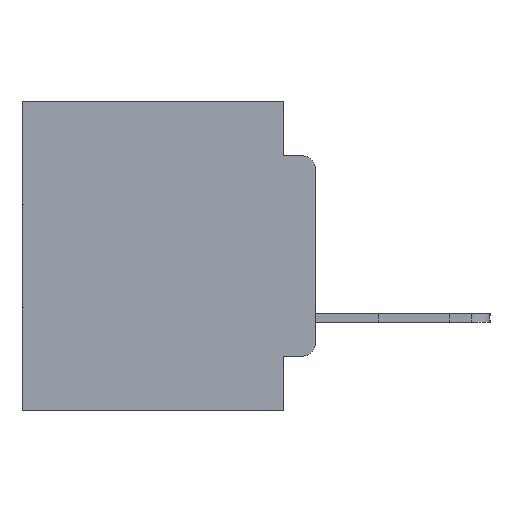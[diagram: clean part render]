
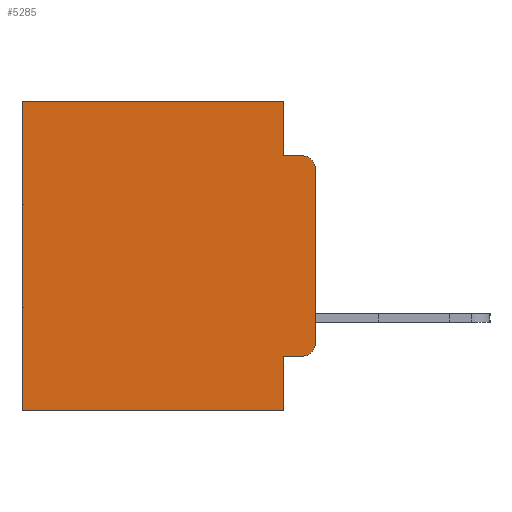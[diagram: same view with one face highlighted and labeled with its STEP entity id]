
A CAD part, left-side view. The second image highlights one B-rep face of the part: STEP entity #5285.
In plain terms, the highlighted planar face has unit normal (-1, 0, 0).
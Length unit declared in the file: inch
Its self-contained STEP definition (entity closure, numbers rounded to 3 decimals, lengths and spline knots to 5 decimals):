
#695 = VECTOR ( 'NONE', #17822, 39.37008 ) ;
#1607 = VERTEX_POINT ( 'NONE', #16577 ) ;
#1611 = CARTESIAN_POINT ( 'NONE',  ( 0.298, 0., 0. ) ) ;
#1712 = CARTESIAN_POINT ( 'NONE',  ( 0.298, 0., 0. ) ) ;
#1968 = LINE ( 'NONE', #10128, #19209 ) ;
#2167 = AXIS2_PLACEMENT_3D ( 'NONE', #1712, #5788, #24165 ) ;
#2727 = CARTESIAN_POINT ( 'NONE',  ( 0.298, 0.02, -0.3915 ) ) ;
#2819 = EDGE_CURVE ( 'NONE', #10604, #18837, #4257, .T. ) ;
#2824 = VERTEX_POINT ( 'NONE', #26158 ) ;
#3047 = CARTESIAN_POINT ( 'NONE',  ( 0.298, 0.051, -0.0885 ) ) ;
#3328 = ORIENTED_EDGE ( 'NONE', *, *, #24447, .F. ) ;
#3439 = VERTEX_POINT ( 'NONE', #17185 ) ;
#4044 = ORIENTED_EDGE ( 'NONE', *, *, #14340, .T. ) ;
#4171 = VERTEX_POINT ( 'NONE', #11172 ) ;
#4222 = FACE_OUTER_BOUND ( 'NONE', #17261, .T. ) ;
#4257 = LINE ( 'NONE', #1611, #21324 ) ;
#4798 = CARTESIAN_POINT ( 'NONE',  ( 0.298, 0.051, 0. ) ) ;
#5040 = DIRECTION ( 'NONE',  ( 0., 0., -1. ) ) ;
#5285 = ADVANCED_FACE ( 'NONE', ( #4222 ), #24320, .F. ) ;
#5398 = CARTESIAN_POINT ( 'NONE',  ( 0.298, 0., -0.1085 ) ) ;
#5788 = DIRECTION ( 'NONE',  ( 1., 0., 0. ) ) ;
#5996 = CIRCLE ( 'NONE', #6770, 0.02 ) ;
#6364 = DIRECTION ( 'NONE',  ( 0., 0., -1. ) ) ;
#6633 = DIRECTION ( 'NONE',  ( -1., 0., 0. ) ) ;
#6770 = AXIS2_PLACEMENT_3D ( 'NONE', #2727, #18402, #5040 ) ;
#7661 = DIRECTION ( 'NONE',  ( 0., -1., 0. ) ) ;
#8198 = DIRECTION ( 'NONE',  ( 0., 0., -1. ) ) ;
#9285 = VERTEX_POINT ( 'NONE', #15529 ) ;
#9409 = CARTESIAN_POINT ( 'NONE',  ( 0.298, 0.473, 0. ) ) ;
#10128 = CARTESIAN_POINT ( 'NONE',  ( 0.298, 0., 0. ) ) ;
#10375 = ORIENTED_EDGE ( 'NONE', *, *, #12024, .F. ) ;
#10604 = VERTEX_POINT ( 'NONE', #4798 ) ;
#10689 = VERTEX_POINT ( 'NONE', #5398 ) ;
#10917 = DIRECTION ( 'NONE',  ( 0., 1., 0. ) ) ;
#11079 = ORIENTED_EDGE ( 'NONE', *, *, #24829, .F. ) ;
#11172 = CARTESIAN_POINT ( 'NONE',  ( 0.298, 0.051, -0.5 ) ) ;
#11578 = LINE ( 'NONE', #18647, #16091 ) ;
#12024 = EDGE_CURVE ( 'NONE', #10689, #16149, #1968, .T. ) ;
#12135 = LINE ( 'NONE', #13140, #16666 ) ;
#12401 = DIRECTION ( 'NONE',  ( 0., 0., -1. ) ) ;
#12491 = ORIENTED_EDGE ( 'NONE', *, *, #18992, .F. ) ;
#12749 = CARTESIAN_POINT ( 'NONE',  ( 0.298, 0., -0.3915 ) ) ;
#13140 = CARTESIAN_POINT ( 'NONE',  ( 0.298, 0., -0.5 ) ) ;
#13609 = EDGE_CURVE ( 'NONE', #1607, #16149, #5996, .T. ) ;
#14340 = EDGE_CURVE ( 'NONE', #2824, #1607, #11578, .T. ) ;
#14456 = LINE ( 'NONE', #21890, #25434 ) ;
#14567 = ORIENTED_EDGE ( 'NONE', *, *, #17510, .T. ) ;
#15175 = DIRECTION ( 'NONE',  ( 0., 1., 0. ) ) ;
#15529 = CARTESIAN_POINT ( 'NONE',  ( 0.298, 0.02, -0.0885 ) ) ;
#15608 = CARTESIAN_POINT ( 'NONE',  ( 0.298, 0.473, 0. ) ) ;
#16091 = VECTOR ( 'NONE', #20752, 39.37008 ) ;
#16149 = VERTEX_POINT ( 'NONE', #12749 ) ;
#16319 = ORIENTED_EDGE ( 'NONE', *, *, #21419, .T. ) ;
#16577 = CARTESIAN_POINT ( 'NONE',  ( 0.298, 0.02, -0.4115 ) ) ;
#16666 = VECTOR ( 'NONE', #10917, 39.37008 ) ;
#16837 = CIRCLE ( 'NONE', #24294, 0.02 ) ;
#17185 = CARTESIAN_POINT ( 'NONE',  ( 0.298, 0.051, -0.0885 ) ) ;
#17261 = EDGE_LOOP ( 'NONE', ( #10375, #16319, #11079, #12491, #19062, #14567, #3328, #26865, #4044, #27561 ) ) ;
#17510 = EDGE_CURVE ( 'NONE', #18837, #26574, #23807, .T. ) ;
#17822 = DIRECTION ( 'NONE',  ( 0., 0., -1. ) ) ;
#17885 = EDGE_CURVE ( 'NONE', #2824, #4171, #27167, .T. ) ;
#18402 = DIRECTION ( 'NONE',  ( -1., 0., 0. ) ) ;
#18647 = CARTESIAN_POINT ( 'NONE',  ( 0.298, 0.051, -0.4115 ) ) ;
#18837 = VERTEX_POINT ( 'NONE', #9409 ) ;
#18992 = EDGE_CURVE ( 'NONE', #10604, #3439, #14456, .T. ) ;
#19062 = ORIENTED_EDGE ( 'NONE', *, *, #2819, .T. ) ;
#19209 = VECTOR ( 'NONE', #12401, 39.37008 ) ;
#19936 = CARTESIAN_POINT ( 'NONE',  ( 0.298, 0.02, -0.1085 ) ) ;
#20014 = VECTOR ( 'NONE', #8198, 39.37008 ) ;
#20752 = DIRECTION ( 'NONE',  ( 0., -1., 0. ) ) ;
#20908 = CARTESIAN_POINT ( 'NONE',  ( 0.298, 0.473, -0.5 ) ) ;
#21324 = VECTOR ( 'NONE', #15175, 39.37008 ) ;
#21419 = EDGE_CURVE ( 'NONE', #10689, #9285, #16837, .T. ) ;
#21440 = CARTESIAN_POINT ( 'NONE',  ( 0.298, 0.051, 0. ) ) ;
#21890 = CARTESIAN_POINT ( 'NONE',  ( 0.298, 0.051, 0. ) ) ;
#22146 = DIRECTION ( 'NONE',  ( 0., 0., -1. ) ) ;
#23122 = VECTOR ( 'NONE', #7661, 39.37008 ) ;
#23807 = LINE ( 'NONE', #15608, #695 ) ;
#24165 = DIRECTION ( 'NONE',  ( 0., 0., -1. ) ) ;
#24294 = AXIS2_PLACEMENT_3D ( 'NONE', #19936, #6633, #22146 ) ;
#24320 = PLANE ( 'NONE',  #2167 ) ;
#24447 = EDGE_CURVE ( 'NONE', #4171, #26574, #12135, .T. ) ;
#24829 = EDGE_CURVE ( 'NONE', #3439, #9285, #28839, .T. ) ;
#25434 = VECTOR ( 'NONE', #6364, 39.37008 ) ;
#26158 = CARTESIAN_POINT ( 'NONE',  ( 0.298, 0.051, -0.4115 ) ) ;
#26574 = VERTEX_POINT ( 'NONE', #20908 ) ;
#26865 = ORIENTED_EDGE ( 'NONE', *, *, #17885, .F. ) ;
#27167 = LINE ( 'NONE', #21440, #20014 ) ;
#27561 = ORIENTED_EDGE ( 'NONE', *, *, #13609, .T. ) ;
#28839 = LINE ( 'NONE', #3047, #23122 ) ;
